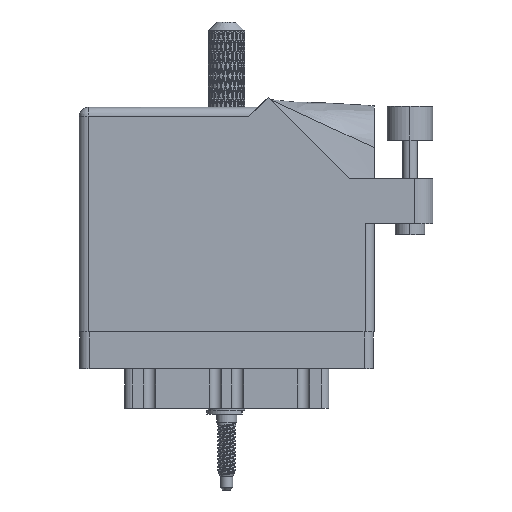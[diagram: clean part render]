
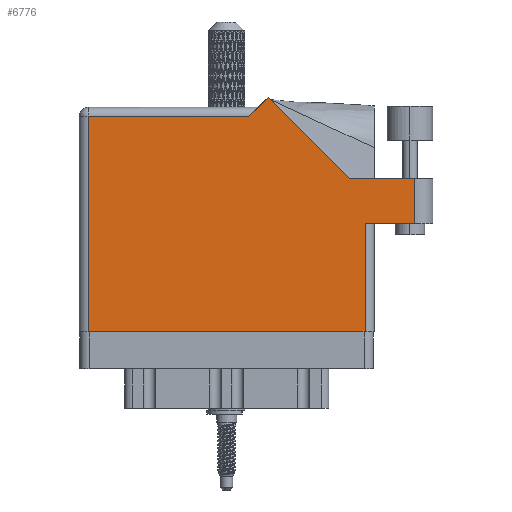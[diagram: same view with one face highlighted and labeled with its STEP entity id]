
A CAD part, front view. The second image highlights one B-rep face of the part: STEP entity #6776.
In plain terms, the highlighted face is planar.
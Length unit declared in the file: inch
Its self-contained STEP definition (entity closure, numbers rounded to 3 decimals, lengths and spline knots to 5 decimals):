
#2081 = LINE ( 'NONE', #71875, #80694 ) ;
#2885 = CARTESIAN_POINT ( 'NONE',  ( 2.01, 0.737, 0. ) ) ;
#4503 = EDGE_CURVE ( 'NONE', #33098, #49268, #99403, .T. ) ;
#5185 = VERTEX_POINT ( 'NONE', #88251 ) ;
#6610 = DIRECTION ( 'NONE',  ( -1., 0., 0. ) ) ;
#6776 = ADVANCED_FACE ( 'NONE', ( #34674 ), #50438, .F. ) ;
#6818 = EDGE_LOOP ( 'NONE', ( #100381, #58673, #51335, #46323, #8420, #79839, #59721, #24970, #72595 ) ) ;
#7499 = CARTESIAN_POINT ( 'NONE',  ( 1.948, 0.737, 0. ) ) ;
#8201 = LINE ( 'NONE', #53535, #91214 ) ;
#8420 = ORIENTED_EDGE ( 'NONE', *, *, #60709, .T. ) ;
#13908 = LINE ( 'NONE', #44999, #72518 ) ;
#14239 = CARTESIAN_POINT ( 'NONE',  ( 0., 1.468, 0. ) ) ;
#16405 = EDGE_CURVE ( 'NONE', #41836, #42615, #2081, .T. ) ;
#16898 = LINE ( 'NONE', #47986, #61161 ) ;
#21602 = AXIS2_PLACEMENT_3D ( 'NONE', #58112, #59631, #59117 ) ;
#24970 = ORIENTED_EDGE ( 'NONE', *, *, #16405, .T. ) ;
#25316 = CARTESIAN_POINT ( 'NONE',  ( 1.84442, 1.044, 0. ) ) ;
#26915 = DIRECTION ( 'NONE',  ( 0., 1., 0. ) ) ;
#29220 = DIRECTION ( 'NONE',  ( 0., 1., 0. ) ) ;
#32858 = VECTOR ( 'NONE', #75529, 39.37008 ) ;
#33098 = VERTEX_POINT ( 'NONE', #25316 ) ;
#34674 = FACE_OUTER_BOUND ( 'NONE', #6818, .T. ) ;
#35766 = CARTESIAN_POINT ( 'NONE',  ( 1.84442, 1.044, 0. ) ) ;
#36254 = EDGE_CURVE ( 'NONE', #52427, #47853, #95069, .T. ) ;
#37026 = CARTESIAN_POINT ( 'NONE',  ( 1.948, 0., 0. ) ) ;
#37181 = LINE ( 'NONE', #14239, #84841 ) ;
#40298 = VECTOR ( 'NONE', #88435, 39.37008 ) ;
#40855 = VECTOR ( 'NONE', #29220, 39.37008 ) ;
#41836 = VERTEX_POINT ( 'NONE', #52281 ) ;
#42615 = VERTEX_POINT ( 'NONE', #37026 ) ;
#44999 = CARTESIAN_POINT ( 'NONE',  ( 2.41, 1.044, 0. ) ) ;
#46323 = ORIENTED_EDGE ( 'NONE', *, *, #4503, .T. ) ;
#46831 = VECTOR ( 'NONE', #26915, 39.37008 ) ;
#46891 = CARTESIAN_POINT ( 'NONE',  ( 2.285, 0.737, 0. ) ) ;
#46943 = DIRECTION ( 'NONE',  ( -0.707, -0.707, 0. ) ) ;
#47853 = VERTEX_POINT ( 'NONE', #46891 ) ;
#47986 = CARTESIAN_POINT ( 'NONE',  ( 0.062, 0., 0. ) ) ;
#49268 = VERTEX_POINT ( 'NONE', #69085 ) ;
#50314 = LINE ( 'NONE', #51843, #46831 ) ;
#50438 = PLANE ( 'NONE',  #21602 ) ;
#51335 = ORIENTED_EDGE ( 'NONE', *, *, #53728, .T. ) ;
#51843 = CARTESIAN_POINT ( 'NONE',  ( 2.285, 1.044, 0. ) ) ;
#52281 = CARTESIAN_POINT ( 'NONE',  ( 0.062, 0., 0. ) ) ;
#52427 = VERTEX_POINT ( 'NONE', #7499 ) ;
#53338 = CARTESIAN_POINT ( 'NONE',  ( 1.155, 1.468, 0. ) ) ;
#53535 = CARTESIAN_POINT ( 'NONE',  ( 1.217, 1.53, 0. ) ) ;
#53728 = EDGE_CURVE ( 'NONE', #5185, #33098, #13908, .T. ) ;
#58112 = CARTESIAN_POINT ( 'NONE',  ( 0., 1.53, 0. ) ) ;
#58673 = ORIENTED_EDGE ( 'NONE', *, *, #89574, .T. ) ;
#59117 = DIRECTION ( 'NONE',  ( -1., 0., 0. ) ) ;
#59631 = DIRECTION ( 'NONE',  ( 0., 0., -1. ) ) ;
#59721 = ORIENTED_EDGE ( 'NONE', *, *, #84135, .T. ) ;
#60709 = EDGE_CURVE ( 'NONE', #49268, #79673, #8201, .T. ) ;
#61161 = VECTOR ( 'NONE', #85706, 39.37008 ) ;
#62319 = EDGE_CURVE ( 'NONE', #79673, #72993, #37181, .T. ) ;
#64731 = DIRECTION ( 'NONE',  ( 1., 0., 0. ) ) ;
#67467 = CARTESIAN_POINT ( 'NONE',  ( 0.062, 1.468, 0. ) ) ;
#68882 = EDGE_CURVE ( 'NONE', #42615, #52427, #98497, .T. ) ;
#69085 = CARTESIAN_POINT ( 'NONE',  ( 1.28771, 1.60071, 0. ) ) ;
#69928 = DIRECTION ( 'NONE',  ( -1., 0., 0. ) ) ;
#71875 = CARTESIAN_POINT ( 'NONE',  ( 0., 0., 0. ) ) ;
#72518 = VECTOR ( 'NONE', #69928, 39.37008 ) ;
#72595 = ORIENTED_EDGE ( 'NONE', *, *, #68882, .T. ) ;
#72993 = VERTEX_POINT ( 'NONE', #67467 ) ;
#73599 = CARTESIAN_POINT ( 'NONE',  ( 1.948, 0.737, 0. ) ) ;
#75529 = DIRECTION ( 'NONE',  ( -0.707, 0.707, 0. ) ) ;
#79673 = VERTEX_POINT ( 'NONE', #53338 ) ;
#79839 = ORIENTED_EDGE ( 'NONE', *, *, #62319, .T. ) ;
#80694 = VECTOR ( 'NONE', #64731, 39.37008 ) ;
#84135 = EDGE_CURVE ( 'NONE', #72993, #41836, #16898, .T. ) ;
#84841 = VECTOR ( 'NONE', #6610, 39.37008 ) ;
#85706 = DIRECTION ( 'NONE',  ( 0., -1., 0. ) ) ;
#88251 = CARTESIAN_POINT ( 'NONE',  ( 2.285, 1.044, 0. ) ) ;
#88435 = DIRECTION ( 'NONE',  ( 1., 0., 0. ) ) ;
#89574 = EDGE_CURVE ( 'NONE', #47853, #5185, #50314, .T. ) ;
#91214 = VECTOR ( 'NONE', #46943, 39.37008 ) ;
#95069 = LINE ( 'NONE', #2885, #40298 ) ;
#98497 = LINE ( 'NONE', #73599, #40855 ) ;
#99403 = LINE ( 'NONE', #35766, #32858 ) ;
#100381 = ORIENTED_EDGE ( 'NONE', *, *, #36254, .T. ) ;
